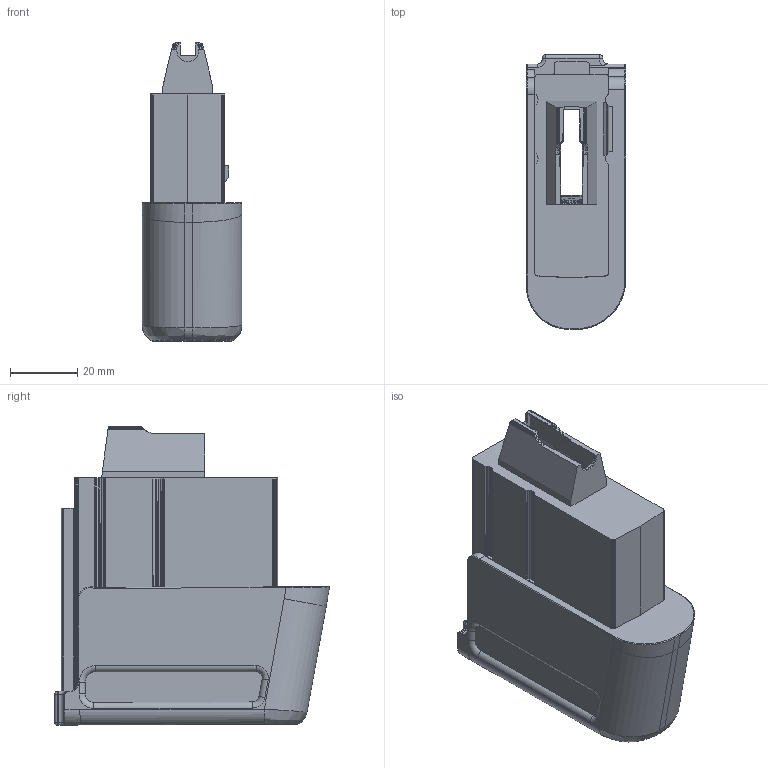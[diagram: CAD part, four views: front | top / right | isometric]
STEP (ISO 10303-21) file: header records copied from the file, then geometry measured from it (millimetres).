
FILE_DESCRIPTION(/* description */ (''),/* implementation_level */ '2;1');
FILE_NAME(/* name */ 'SG22 Short Magazine.step',/* time_stamp */ '2021-01-18T14:17:04-07:00',/* author */ (''),/* organization */ (''),/* preprocessor_version */ 'ST-DEVELOPER v18.1',/* originating_system */ 'Autodesk Translation Framework v9.7.1.1290',/* authorisation */ '');
FILE_SCHEMA (('AUTOMOTIVE_DESIGN { 1 0 10303 214 3 1 1 }'));
Length unit declared in the file: inch
Products named in the file (1): Space Gun Beta Ready
Bounding box: 29.62 x 81.84 x 88.76 mm (x, y, z)
Volume: 96580.9 mm3; surface area: 30684.9 mm2
Topology: 1 solids, 6 shells, 2207 faces, 4250 edges, 2055 vertices
Faces by surface type: plane 2121, cylinder 52, torus 19, bspline 13, sphere 2
Entity records: 52316 total; most frequent: CARTESIAN_POINT 9200, DIRECTION 8737, ORIENTED_EDGE 8500, EDGE_CURVE 4250, LINE 4093, VECTOR 4093, AXIS2_PLACEMENT_3D 2322, EDGE_LOOP 2213
